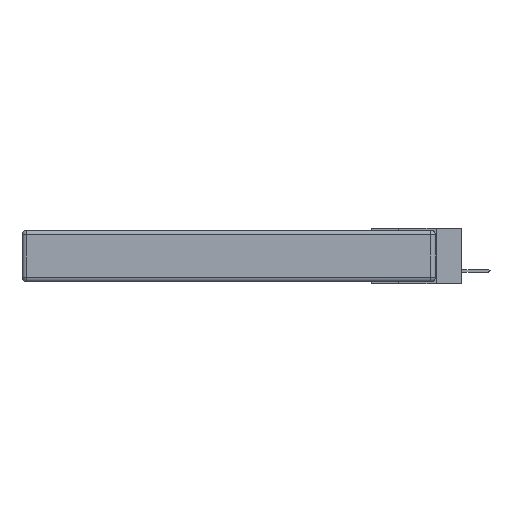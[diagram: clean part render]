
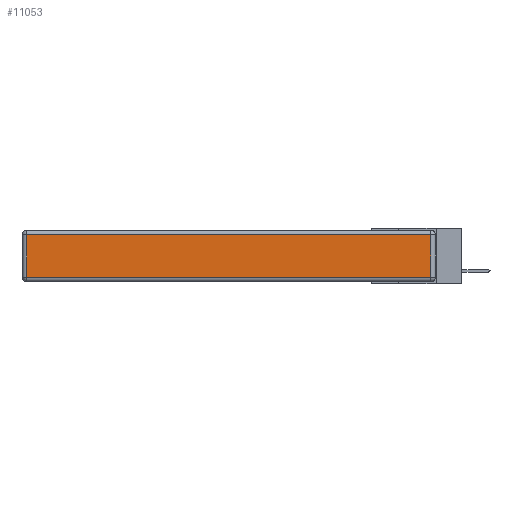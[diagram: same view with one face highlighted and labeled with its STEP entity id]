
A CAD part, left-side view. The second image highlights one B-rep face of the part: STEP entity #11053.
In plain terms, the highlighted planar face has unit normal (-1, 0, 0).
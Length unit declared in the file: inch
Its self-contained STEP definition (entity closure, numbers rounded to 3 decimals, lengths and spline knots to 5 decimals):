
#1553 = EDGE_LOOP ( 'NONE', ( #2578, #18849, #8048, #13518 ) ) ;
#2578 = ORIENTED_EDGE ( 'NONE', *, *, #5969, .T. ) ;
#3214 = VERTEX_POINT ( 'NONE', #11562 ) ;
#3679 = CARTESIAN_POINT ( 'NONE',  ( 0., 0.03, -0.343 ) ) ;
#4745 = VECTOR ( 'NONE', #14705, 39.37008 ) ;
#5585 = DIRECTION ( 'NONE',  ( -1., 0., 0. ) ) ;
#5969 = EDGE_CURVE ( 'NONE', #23262, #23746, #6825, .T. ) ;
#5989 = FACE_OUTER_BOUND ( 'NONE', #1553, .T. ) ;
#6092 = CARTESIAN_POINT ( 'NONE',  ( 0., 2.72, -0.313 ) ) ;
#6226 = EDGE_CURVE ( 'NONE', #23746, #11571, #14800, .T. ) ;
#6825 = LINE ( 'NONE', #22539, #15541 ) ;
#8048 = ORIENTED_EDGE ( 'NONE', *, *, #27755, .T. ) ;
#8315 = EDGE_CURVE ( 'NONE', #3214, #23262, #25747, .T. ) ;
#9207 = CARTESIAN_POINT ( 'NONE',  ( 0., 2.75, -0.03 ) ) ;
#11053 = ADVANCED_FACE ( 'NONE', ( #5989 ), #16647, .T. ) ;
#11562 = CARTESIAN_POINT ( 'NONE',  ( 0., 2.72, -0.03 ) ) ;
#11571 = VERTEX_POINT ( 'NONE', #12181 ) ;
#12181 = CARTESIAN_POINT ( 'NONE',  ( 0., 0.03, -0.03 ) ) ;
#13278 = VECTOR ( 'NONE', #24835, 39.37008 ) ;
#13518 = ORIENTED_EDGE ( 'NONE', *, *, #8315, .T. ) ;
#13618 = CARTESIAN_POINT ( 'NONE',  ( 0., 2.72, -0.343 ) ) ;
#14705 = DIRECTION ( 'NONE',  ( 0., 0., 1. ) ) ;
#14800 = LINE ( 'NONE', #3679, #4745 ) ;
#15541 = VECTOR ( 'NONE', #26729, 39.37008 ) ;
#16647 = PLANE ( 'NONE',  #17149 ) ;
#17149 = AXIS2_PLACEMENT_3D ( 'NONE', #18869, #5585, #21079 ) ;
#18331 = DIRECTION ( 'NONE',  ( 0., 1., 0. ) ) ;
#18849 = ORIENTED_EDGE ( 'NONE', *, *, #6226, .T. ) ;
#18869 = CARTESIAN_POINT ( 'NONE',  ( 0., 0., -0.343 ) ) ;
#21079 = DIRECTION ( 'NONE',  ( 0., 0., 1. ) ) ;
#21135 = CARTESIAN_POINT ( 'NONE',  ( 0., 0.03, -0.313 ) ) ;
#22539 = CARTESIAN_POINT ( 'NONE',  ( 0., 0., -0.313 ) ) ;
#23262 = VERTEX_POINT ( 'NONE', #6092 ) ;
#23746 = VERTEX_POINT ( 'NONE', #21135 ) ;
#24835 = DIRECTION ( 'NONE',  ( 0., 0., -1. ) ) ;
#25747 = LINE ( 'NONE', #13618, #13278 ) ;
#26425 = VECTOR ( 'NONE', #18331, 39.37008 ) ;
#26729 = DIRECTION ( 'NONE',  ( 0., -1., 0. ) ) ;
#26751 = LINE ( 'NONE', #9207, #26425 ) ;
#27755 = EDGE_CURVE ( 'NONE', #11571, #3214, #26751, .T. ) ;
